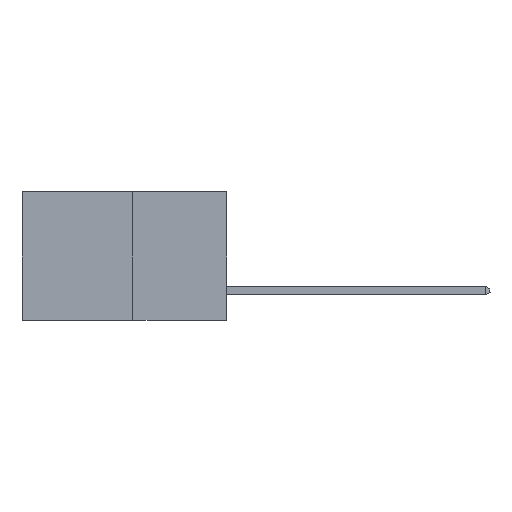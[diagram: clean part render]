
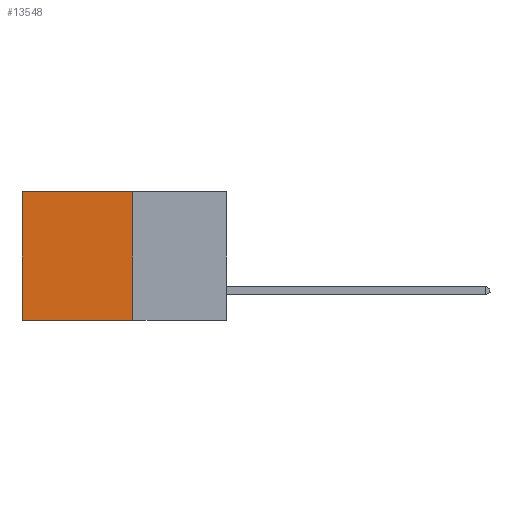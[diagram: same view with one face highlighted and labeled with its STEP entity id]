
A CAD part, left-side view. The second image highlights one B-rep face of the part: STEP entity #13548.
In plain terms, the highlighted planar face has unit normal (-1, 0, 0).
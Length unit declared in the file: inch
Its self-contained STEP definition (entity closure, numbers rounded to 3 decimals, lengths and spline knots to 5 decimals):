
#58 = DIRECTION ( 'NONE',  ( 1., 0., 0. ) ) ;
#1224 = VERTEX_POINT ( 'NONE', #11895 ) ;
#1354 = DIRECTION ( 'NONE',  ( 0., 0., -1. ) ) ;
#1647 = VERTEX_POINT ( 'NONE', #11724 ) ;
#2541 = CARTESIAN_POINT ( 'NONE',  ( 0.277, 0.27, 0. ) ) ;
#3068 = EDGE_LOOP ( 'NONE', ( #10323, #7469, #16258, #3930 ) ) ;
#3930 = ORIENTED_EDGE ( 'NONE', *, *, #6145, .T. ) ;
#4808 = EDGE_CURVE ( 'NONE', #1647, #10297, #6753, .T. ) ;
#5045 = VERTEX_POINT ( 'NONE', #17123 ) ;
#6145 = EDGE_CURVE ( 'NONE', #5045, #1224, #10267, .T. ) ;
#6569 = VECTOR ( 'NONE', #14161, 39.37008 ) ;
#6753 = LINE ( 'NONE', #13571, #13160 ) ;
#7469 = ORIENTED_EDGE ( 'NONE', *, *, #4808, .F. ) ;
#8190 = CARTESIAN_POINT ( 'NONE',  ( 0.277, 0.27, -0.37 ) ) ;
#8268 = DIRECTION ( 'NONE',  ( 0., 0., -1. ) ) ;
#8354 = CARTESIAN_POINT ( 'NONE',  ( 0.277, 0.27, -0.37 ) ) ;
#8814 = FACE_OUTER_BOUND ( 'NONE', #3068, .T. ) ;
#9704 = CARTESIAN_POINT ( 'NONE',  ( 0.277, 0.59, -0.37 ) ) ;
#9793 = DIRECTION ( 'NONE',  ( 0., 0., -1. ) ) ;
#9962 = CARTESIAN_POINT ( 'NONE',  ( 0.277, 0.59, -0.37 ) ) ;
#10267 = LINE ( 'NONE', #2541, #6569 ) ;
#10297 = VERTEX_POINT ( 'NONE', #9962 ) ;
#10323 = ORIENTED_EDGE ( 'NONE', *, *, #14143, .T. ) ;
#10807 = EDGE_CURVE ( 'NONE', #5045, #1647, #11983, .T. ) ;
#11724 = CARTESIAN_POINT ( 'NONE',  ( 0.277, 0.27, -0.37 ) ) ;
#11732 = DIRECTION ( 'NONE',  ( 0., 1., 0. ) ) ;
#11895 = CARTESIAN_POINT ( 'NONE',  ( 0.277, 0.59, 0. ) ) ;
#11983 = LINE ( 'NONE', #8190, #15854 ) ;
#12187 = LINE ( 'NONE', #9704, #16458 ) ;
#13160 = VECTOR ( 'NONE', #11732, 39.37008 ) ;
#13548 = ADVANCED_FACE ( 'NONE', ( #8814 ), #16323, .F. ) ;
#13571 = CARTESIAN_POINT ( 'NONE',  ( 0.277, 0.27, -0.37 ) ) ;
#14143 = EDGE_CURVE ( 'NONE', #1224, #10297, #12187, .T. ) ;
#14161 = DIRECTION ( 'NONE',  ( 0., 1., 0. ) ) ;
#15854 = VECTOR ( 'NONE', #1354, 39.37008 ) ;
#16258 = ORIENTED_EDGE ( 'NONE', *, *, #10807, .F. ) ;
#16323 = PLANE ( 'NONE',  #17497 ) ;
#16458 = VECTOR ( 'NONE', #8268, 39.37008 ) ;
#17123 = CARTESIAN_POINT ( 'NONE',  ( 0.277, 0.27, 0. ) ) ;
#17497 = AXIS2_PLACEMENT_3D ( 'NONE', #8354, #58, #9793 ) ;
